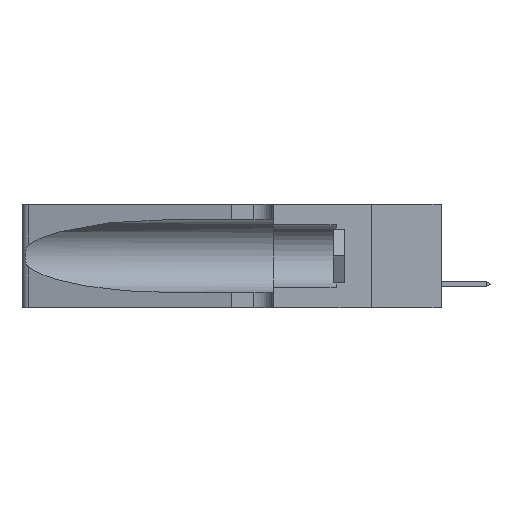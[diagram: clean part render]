
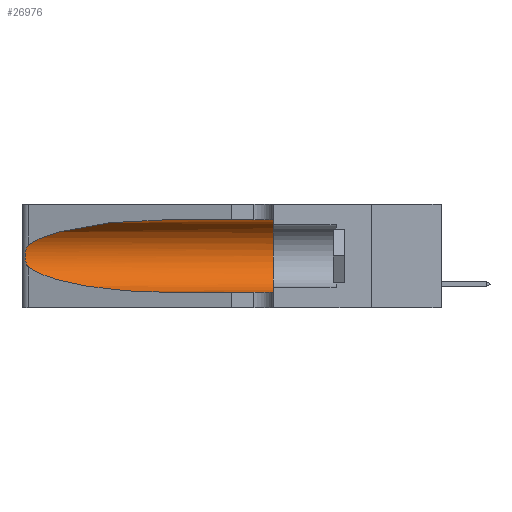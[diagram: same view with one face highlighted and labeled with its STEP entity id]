
A CAD part, left-side view. The second image highlights one B-rep face of the part: STEP entity #26976.
In plain terms, the highlighted cylindrical face has radius 3.308 mm (diameter 6.617 mm), a partial arc.
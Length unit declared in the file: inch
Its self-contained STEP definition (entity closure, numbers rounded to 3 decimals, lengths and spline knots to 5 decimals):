
#129 = ORIENTED_EDGE ( 'NONE', *, *, #2716, .T. ) ;
#402 = CARTESIAN_POINT ( 'NONE',  ( 0.18966, 0.96281, 0.05475 ) ) ;
#1547 = DIRECTION ( 'NONE',  ( 0., 1., 0. ) ) ;
#2563 = CARTESIAN_POINT ( 'NONE',  ( 0.25639, 1.23184, 0.21858 ) ) ;
#2716 = EDGE_CURVE ( 'NONE', #18275, #28362, #28708, .T. ) ;
#2824 = VERTEX_POINT ( 'NONE', #12511 ) ;
#3423 = EDGE_CURVE ( 'NONE', #11118, #2824, #22571, .T. ) ;
#3834 = DIRECTION ( 'NONE',  ( 0., -1., 0. ) ) ;
#4712 = CARTESIAN_POINT ( 'NONE',  ( 0.1305, 1.61858, 0.31525 ) ) ;
#4858 = EDGE_CURVE ( 'NONE', #11118, #15997, #10481, .T. ) ;
#5153 = CARTESIAN_POINT ( 'NONE',  ( 0.25787, 1.23484, 0.2124 ) ) ;
#5699 = CARTESIAN_POINT ( 'NONE',  ( 0.26075, 1.23896, 0.19203 ) ) ;
#6842 = ORIENTED_EDGE ( 'NONE', *, *, #22439, .T. ) ;
#8298 = ORIENTED_EDGE ( 'NONE', *, *, #3423, .F. ) ;
#8488 = CARTESIAN_POINT ( 'NONE',  ( 0.25487, 1.22718, 0.22369 ) ) ;
#9045 = CARTESIAN_POINT ( 'NONE',  ( 0.1305, 1.61858, 0.05475 ) ) ;
#9169 = DIRECTION ( 'NONE',  ( 0., -1., 0. ) ) ;
#9263 = ORIENTED_EDGE ( 'NONE', *, *, #16658, .F. ) ;
#9732 = DIRECTION ( 'NONE',  ( 0., 0., -1. ) ) ;
#10141 = CIRCLE ( 'NONE', #28518, 0.13025 ) ;
#10481 =( BOUNDED_CURVE ( )  B_SPLINE_CURVE ( 3, ( #15255, #28478, #17418, #38552 ),
 .UNSPECIFIED., .F., .T. ) 
 B_SPLINE_CURVE_WITH_KNOTS ( ( 4, 4 ),
 ( 1.5708, 2.84003 ),
 .UNSPECIFIED. ) 
 CURVE ( )  GEOMETRIC_REPRESENTATION_ITEM ( )  RATIONAL_B_SPLINE_CURVE ( ( 1., 0.87, 0.87, 1. ) ) 
 REPRESENTATION_ITEM ( '' )  );
#11118 = VERTEX_POINT ( 'NONE', #38325 ) ;
#11132 = CARTESIAN_POINT ( 'NONE',  ( 0.25854, 1.2359, 0.20912 ) ) ;
#11522 = CARTESIAN_POINT ( 'NONE',  ( 0.25555, 1.22994, 0.2215 ) ) ;
#12014 = VECTOR ( 'NONE', #9169, 39.37008 ) ;
#12511 = CARTESIAN_POINT ( 'NONE',  ( 0.1305, 0.35, 0.31525 ) ) ;
#13922 = CARTESIAN_POINT ( 'NONE',  ( 0.1305, 0.72297, 0.05475 ) ) ;
#14314 = CARTESIAN_POINT ( 'NONE',  ( 0.25856, 1.23593, 0.16098 ) ) ;
#14453 = CARTESIAN_POINT ( 'NONE',  ( 0.26018, 1.23835, 0.19895 ) ) ;
#14560 = FACE_OUTER_BOUND ( 'NONE', #27438, .T. ) ;
#14589 = CARTESIAN_POINT ( 'NONE',  ( 0.25639, 1.23186, 0.15144 ) ) ;
#15255 = CARTESIAN_POINT ( 'NONE',  ( 0.1305, 0.72297, 0.31525 ) ) ;
#15424 = VECTOR ( 'NONE', #29922, 39.37008 ) ;
#15997 = VERTEX_POINT ( 'NONE', #31813 ) ;
#16658 = EDGE_CURVE ( 'NONE', #2824, #17716, #10141, .T. ) ;
#17243 = CARTESIAN_POINT ( 'NONE',  ( 0.25555, 1.22993, 0.14849 ) ) ;
#17385 = CARTESIAN_POINT ( 'NONE',  ( 0.25789, 1.23486, 0.15765 ) ) ;
#17418 = CARTESIAN_POINT ( 'NONE',  ( 0.2373, 1.15595, 0.28018 ) ) ;
#17716 = VERTEX_POINT ( 'NONE', #22811 ) ;
#18275 = VERTEX_POINT ( 'NONE', #25266 ) ;
#18704 = CARTESIAN_POINT ( 'NONE',  ( 0.25487, 1.22718, 0.14631 ) ) ;
#21607 = CARTESIAN_POINT ( 'NONE',  ( 0.1305, 0.72297, 0.05475 ) ) ;
#22439 = EDGE_CURVE ( 'NONE', #15997, #18275, #34615, .T. ) ;
#22571 = LINE ( 'NONE', #4712, #15424 ) ;
#22811 = CARTESIAN_POINT ( 'NONE',  ( 0.1305, 0.35, 0.05475 ) ) ;
#23246 = AXIS2_PLACEMENT_3D ( 'NONE', #34474, #3834, #9732 ) ;
#23613 = CARTESIAN_POINT ( 'NONE',  ( 0.25487, 1.22718, 0.14631 ) ) ;
#23862 = CARTESIAN_POINT ( 'NONE',  ( 0.26075, 1.23896, 0.178 ) ) ;
#24823 = EDGE_CURVE ( 'NONE', #28362, #17716, #25714, .T. ) ;
#25266 = CARTESIAN_POINT ( 'NONE',  ( 0.25487, 1.22718, 0.14631 ) ) ;
#25714 = LINE ( 'NONE', #9045, #12014 ) ;
#26976 = ADVANCED_FACE ( 'NONE', ( #14560 ), #33976, .F. ) ;
#27438 = EDGE_LOOP ( 'NONE', ( #37045, #6842, #129, #30404, #9263, #8298 ) ) ;
#28217 = CARTESIAN_POINT ( 'NONE',  ( 0.2373, 1.15595, 0.08982 ) ) ;
#28362 = VERTEX_POINT ( 'NONE', #13922 ) ;
#28478 = CARTESIAN_POINT ( 'NONE',  ( 0.18966, 0.96281, 0.31525 ) ) ;
#28518 = AXIS2_PLACEMENT_3D ( 'NONE', #34854, #1547, #28934 ) ;
#28708 =( BOUNDED_CURVE ( )  B_SPLINE_CURVE ( 3, ( #18704, #28217, #402, #21607 ),
 .UNSPECIFIED., .F., .T. ) 
 B_SPLINE_CURVE_WITH_KNOTS ( ( 4, 4 ),
 ( 3.44316, 4.71239 ),
 .UNSPECIFIED. ) 
 CURVE ( )  GEOMETRIC_REPRESENTATION_ITEM ( )  RATIONAL_B_SPLINE_CURVE ( ( 1., 0.87, 0.87, 1. ) ) 
 REPRESENTATION_ITEM ( '' )  );
#28934 = DIRECTION ( 'NONE',  ( 0., 0., 1. ) ) ;
#29922 = DIRECTION ( 'NONE',  ( 0., -1., 0. ) ) ;
#30404 = ORIENTED_EDGE ( 'NONE', *, *, #24823, .T. ) ;
#31813 = CARTESIAN_POINT ( 'NONE',  ( 0.25487, 1.22718, 0.22369 ) ) ;
#32807 = CARTESIAN_POINT ( 'NONE',  ( 0.26017, 1.23833, 0.17102 ) ) ;
#33976 = CYLINDRICAL_SURFACE ( 'NONE', #23246, 0.13025 ) ;
#34474 = CARTESIAN_POINT ( 'NONE',  ( 0.1305, 1.61858, 0.185 ) ) ;
#34615 = B_SPLINE_CURVE_WITH_KNOTS ( 'NONE', 3,
 ( #8488, #11522, #2563, #5153, #11132, #14453, #5699, #23862, #32807, #14314, #17385, #14589, #17243, #23613 ),
 .UNSPECIFIED., .F., .F.,
 ( 4, 2, 2, 2, 2, 2, 4 ),
 ( 0., 0.00027, 0.00053, 0.00107, 0.0016, 0.00187, 0.00214 ),
 .UNSPECIFIED. ) ;
#34854 = CARTESIAN_POINT ( 'NONE',  ( 0.1305, 0.35, 0.185 ) ) ;
#37045 = ORIENTED_EDGE ( 'NONE', *, *, #4858, .T. ) ;
#38325 = CARTESIAN_POINT ( 'NONE',  ( 0.1305, 0.72297, 0.31525 ) ) ;
#38552 = CARTESIAN_POINT ( 'NONE',  ( 0.25487, 1.22718, 0.22369 ) ) ;
